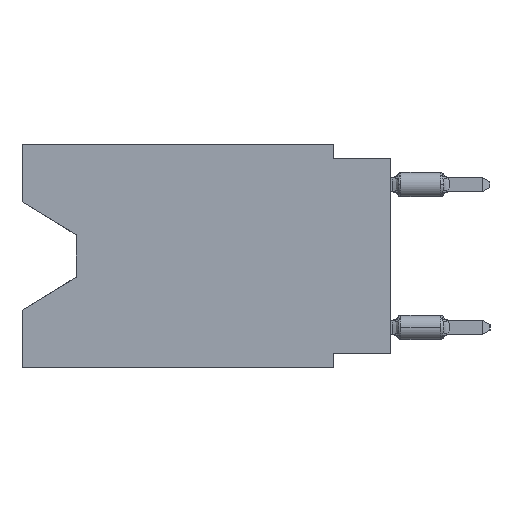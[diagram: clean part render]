
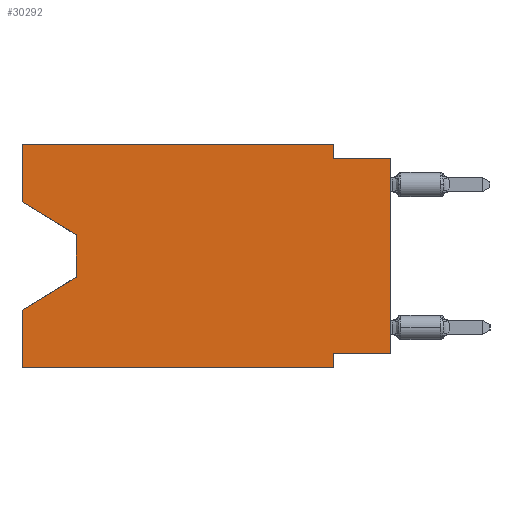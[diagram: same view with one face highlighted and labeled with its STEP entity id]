
A CAD part, left-side view. The second image highlights one B-rep face of the part: STEP entity #30292.
In plain terms, the highlighted planar face has unit normal (-1, 0, 0).
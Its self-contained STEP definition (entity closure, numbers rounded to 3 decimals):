
#991 = LINE ( 'NONE', #21811, #21644 ) ;
#1482 = ORIENTED_EDGE ( 'NONE', *, *, #14173, .T. ) ;
#1871 = DIRECTION ( 'NONE',  ( 0., 0., -1. ) ) ;
#3243 = DIRECTION ( 'NONE',  ( 0., -1., 0. ) ) ;
#3367 = DIRECTION ( 'NONE',  ( 0., -0.855, -0.519 ) ) ;
#3447 = DIRECTION ( 'NONE',  ( 0., 0., -1. ) ) ;
#4051 = ORIENTED_EDGE ( 'NONE', *, *, #46348, .F. ) ;
#4668 = CARTESIAN_POINT ( 'NONE',  ( 0., 16.383, 0. ) ) ;
#6547 = AXIS2_PLACEMENT_3D ( 'NONE', #13371, #32943, #52575 ) ;
#7090 = CARTESIAN_POINT ( 'NONE',  ( 0., 2.54, -9.906 ) ) ;
#7407 = CARTESIAN_POINT ( 'NONE',  ( 0., 2.54, -9.271 ) ) ;
#7524 = VECTOR ( 'NONE', #39296, 1000. ) ;
#7774 = CARTESIAN_POINT ( 'NONE',  ( 0., 0., -0.635 ) ) ;
#8507 = CARTESIAN_POINT ( 'NONE',  ( 0., 16.383, 0. ) ) ;
#8686 = DIRECTION ( 'NONE',  ( 0., 0., -1. ) ) ;
#8801 = ORIENTED_EDGE ( 'NONE', *, *, #48467, .F. ) ;
#8820 = LINE ( 'NONE', #8507, #57815 ) ;
#9546 = VECTOR ( 'NONE', #51994, 1000. ) ;
#12425 = ORIENTED_EDGE ( 'NONE', *, *, #57810, .T. ) ;
#12631 = EDGE_CURVE ( 'NONE', #40886, #53593, #991, .T. ) ;
#12760 = ORIENTED_EDGE ( 'NONE', *, *, #12631, .F. ) ;
#12826 = VECTOR ( 'NONE', #3243, 1000. ) ;
#13003 = VECTOR ( 'NONE', #3447, 1000. ) ;
#13061 = CARTESIAN_POINT ( 'NONE',  ( 0., 2.54, 0. ) ) ;
#13241 = DIRECTION ( 'NONE',  ( 0., -1., 0. ) ) ;
#13290 = LINE ( 'NONE', #31593, #42398 ) ;
#13371 = CARTESIAN_POINT ( 'NONE',  ( 0., 16.383, 0. ) ) ;
#14173 = EDGE_CURVE ( 'NONE', #46764, #54208, #36210, .T. ) ;
#14625 = CARTESIAN_POINT ( 'NONE',  ( 0., 16.383, -9.906 ) ) ;
#14851 = EDGE_CURVE ( 'NONE', #32884, #33874, #24515, .T. ) ;
#15446 = EDGE_CURVE ( 'NONE', #53593, #41782, #31464, .T. ) ;
#16122 = DIRECTION ( 'NONE',  ( 0., 0., 1. ) ) ;
#16149 = CARTESIAN_POINT ( 'NONE',  ( 0., 13.97, -4.013 ) ) ;
#17228 = ORIENTED_EDGE ( 'NONE', *, *, #46191, .T. ) ;
#17297 = CARTESIAN_POINT ( 'NONE',  ( 0., 13.97, -5.893 ) ) ;
#17354 = CARTESIAN_POINT ( 'NONE',  ( 0., 0., -0.635 ) ) ;
#18870 = VECTOR ( 'NONE', #8686, 1000. ) ;
#19195 = ORIENTED_EDGE ( 'NONE', *, *, #15446, .F. ) ;
#19677 = DIRECTION ( 'NONE',  ( 0., 0., 1. ) ) ;
#20243 = EDGE_CURVE ( 'NONE', #55515, #25528, #57066, .T. ) ;
#21310 = VECTOR ( 'NONE', #23874, 1000. ) ;
#21644 = VECTOR ( 'NONE', #41419, 1000. ) ;
#21811 = CARTESIAN_POINT ( 'NONE',  ( 0., 0., -9.271 ) ) ;
#21952 = EDGE_CURVE ( 'NONE', #32884, #41782, #23240, .T. ) ;
#22531 = VERTEX_POINT ( 'NONE', #40388 ) ;
#23240 = LINE ( 'NONE', #43797, #21310 ) ;
#23525 = ORIENTED_EDGE ( 'NONE', *, *, #21952, .T. ) ;
#23526 = VERTEX_POINT ( 'NONE', #35211 ) ;
#23850 = VECTOR ( 'NONE', #1871, 1000. ) ;
#23874 = DIRECTION ( 'NONE',  ( 0., -1., 0. ) ) ;
#23975 = CARTESIAN_POINT ( 'NONE',  ( 0., 2.54, 0. ) ) ;
#24515 = LINE ( 'NONE', #4668, #7524 ) ;
#25528 = VERTEX_POINT ( 'NONE', #41402 ) ;
#26059 = CARTESIAN_POINT ( 'NONE',  ( 0., 0., 0. ) ) ;
#28042 = VERTEX_POINT ( 'NONE', #7774 ) ;
#29685 = EDGE_LOOP ( 'NONE', ( #17228, #1482, #51197, #55167, #23525, #19195, #12760, #12425, #8801, #52961, #56707, #4051 ) ) ;
#30292 = ADVANCED_FACE ( 'NONE', ( #57378 ), #63126, .F. ) ;
#31464 = LINE ( 'NONE', #7090, #18870 ) ;
#31593 = CARTESIAN_POINT ( 'NONE',  ( 0., 16.383, -2.546 ) ) ;
#31701 = CARTESIAN_POINT ( 'NONE',  ( 0., 13.97, -4.013 ) ) ;
#32884 = VERTEX_POINT ( 'NONE', #14625 ) ;
#32943 = DIRECTION ( 'NONE',  ( 1., 0., 0. ) ) ;
#33605 = CARTESIAN_POINT ( 'NONE',  ( 0., 13.97, -5.893 ) ) ;
#33874 = VERTEX_POINT ( 'NONE', #53991 ) ;
#35211 = CARTESIAN_POINT ( 'NONE',  ( 0., 16.383, -2.546 ) ) ;
#36210 = LINE ( 'NONE', #31701, #23850 ) ;
#39296 = DIRECTION ( 'NONE',  ( 0., 0., 1. ) ) ;
#40388 = CARTESIAN_POINT ( 'NONE',  ( 0., 16.383, 0. ) ) ;
#40886 = VERTEX_POINT ( 'NONE', #45241 ) ;
#41402 = CARTESIAN_POINT ( 'NONE',  ( 0., 2.54, -0.635 ) ) ;
#41419 = DIRECTION ( 'NONE',  ( 0., 1., 0. ) ) ;
#41452 = CARTESIAN_POINT ( 'NONE',  ( 0., 2.54, -9.906 ) ) ;
#41513 = CARTESIAN_POINT ( 'NONE',  ( 0., 16.383, 0. ) ) ;
#41782 = VERTEX_POINT ( 'NONE', #41452 ) ;
#42398 = VECTOR ( 'NONE', #3367, 1000. ) ;
#43797 = CARTESIAN_POINT ( 'NONE',  ( 0., 16.383, -9.906 ) ) ;
#44152 = EDGE_CURVE ( 'NONE', #54208, #33874, #61606, .T. ) ;
#44468 = VECTOR ( 'NONE', #16122, 1000. ) ;
#45241 = CARTESIAN_POINT ( 'NONE',  ( 0., 0., -9.271 ) ) ;
#46191 = EDGE_CURVE ( 'NONE', #23526, #46764, #13290, .T. ) ;
#46348 = EDGE_CURVE ( 'NONE', #23526, #22531, #8820, .T. ) ;
#46764 = VERTEX_POINT ( 'NONE', #16149 ) ;
#48094 = EDGE_CURVE ( 'NONE', #22531, #55515, #61741, .T. ) ;
#48467 = EDGE_CURVE ( 'NONE', #25528, #28042, #51736, .T. ) ;
#51197 = ORIENTED_EDGE ( 'NONE', *, *, #44152, .T. ) ;
#51736 = LINE ( 'NONE', #17354, #12826 ) ;
#51994 = DIRECTION ( 'NONE',  ( 0., 0.855, -0.519 ) ) ;
#52575 = DIRECTION ( 'NONE',  ( 0., 0., -1. ) ) ;
#52961 = ORIENTED_EDGE ( 'NONE', *, *, #20243, .F. ) ;
#53593 = VERTEX_POINT ( 'NONE', #7407 ) ;
#53991 = CARTESIAN_POINT ( 'NONE',  ( 0., 16.383, -7.36 ) ) ;
#54208 = VERTEX_POINT ( 'NONE', #33605 ) ;
#55167 = ORIENTED_EDGE ( 'NONE', *, *, #14851, .F. ) ;
#55515 = VERTEX_POINT ( 'NONE', #23975 ) ;
#56707 = ORIENTED_EDGE ( 'NONE', *, *, #48094, .F. ) ;
#57066 = LINE ( 'NONE', #13061, #13003 ) ;
#57378 = FACE_OUTER_BOUND ( 'NONE', #29685, .T. ) ;
#57810 = EDGE_CURVE ( 'NONE', #40886, #28042, #59796, .T. ) ;
#57815 = VECTOR ( 'NONE', #19677, 1000. ) ;
#57943 = VECTOR ( 'NONE', #13241, 1000. ) ;
#59796 = LINE ( 'NONE', #26059, #44468 ) ;
#61606 = LINE ( 'NONE', #17297, #9546 ) ;
#61741 = LINE ( 'NONE', #41513, #57943 ) ;
#63126 = PLANE ( 'NONE',  #6547 ) ;
